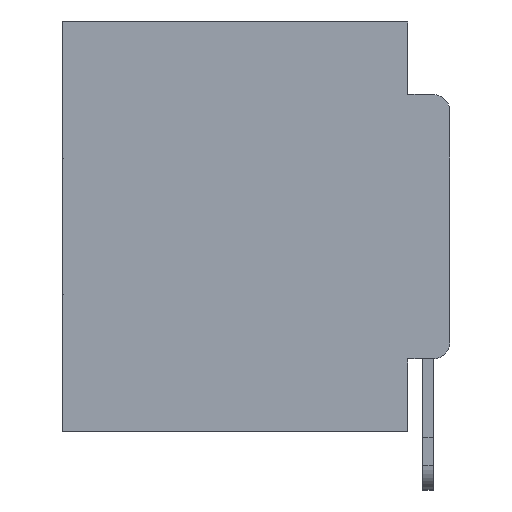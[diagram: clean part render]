
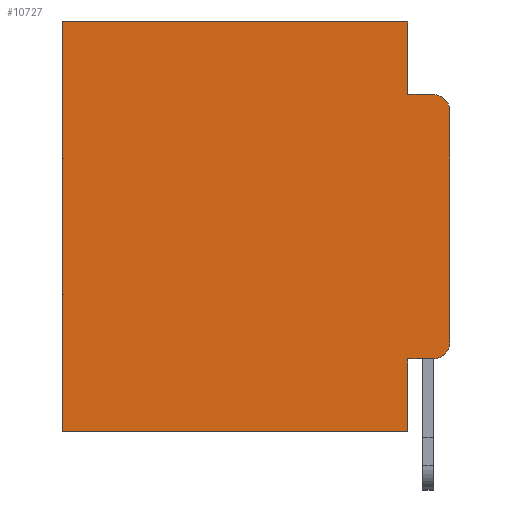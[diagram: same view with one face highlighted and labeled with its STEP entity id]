
A CAD part, left-side view. The second image highlights one B-rep face of the part: STEP entity #10727.
In plain terms, the highlighted planar face has unit normal (-1, 0, 0).
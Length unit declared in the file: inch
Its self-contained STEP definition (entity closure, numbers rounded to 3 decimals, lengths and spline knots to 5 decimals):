
#312 = CARTESIAN_POINT ( 'NONE',  ( 0.298, 0., -0.5 ) ) ;
#399 = EDGE_CURVE ( 'NONE', #8756, #29636, #10669, .T. ) ;
#598 = CARTESIAN_POINT ( 'NONE',  ( 0.298, 0.051, -0.5 ) ) ;
#694 = VERTEX_POINT ( 'NONE', #23454 ) ;
#695 = CARTESIAN_POINT ( 'NONE',  ( 0.298, 0.051, -0.0885 ) ) ;
#1277 = CARTESIAN_POINT ( 'NONE',  ( 0.298, 0.473, 0. ) ) ;
#1932 = CARTESIAN_POINT ( 'NONE',  ( 0.298, 0., -0.3915 ) ) ;
#1965 = ORIENTED_EDGE ( 'NONE', *, *, #18255, .T. ) ;
#2171 = VERTEX_POINT ( 'NONE', #18730 ) ;
#2199 = VERTEX_POINT ( 'NONE', #28101 ) ;
#2334 = ORIENTED_EDGE ( 'NONE', *, *, #22888, .F. ) ;
#2927 = VERTEX_POINT ( 'NONE', #16836 ) ;
#3115 = DIRECTION ( 'NONE',  ( 0., 1., 0. ) ) ;
#3500 = CARTESIAN_POINT ( 'NONE',  ( 0.298, 0.02, -0.3915 ) ) ;
#3688 = CARTESIAN_POINT ( 'NONE',  ( 0.298, 0.02, -0.4115 ) ) ;
#3962 = EDGE_CURVE ( 'NONE', #8756, #24440, #10182, .T. ) ;
#4555 = VECTOR ( 'NONE', #7029, 39.37008 ) ;
#4608 = ORIENTED_EDGE ( 'NONE', *, *, #13509, .F. ) ;
#5207 = DIRECTION ( 'NONE',  ( 0., 1., 0. ) ) ;
#5324 = VECTOR ( 'NONE', #5207, 39.37008 ) ;
#5729 = DIRECTION ( 'NONE',  ( -1., 0., 0. ) ) ;
#6112 = DIRECTION ( 'NONE',  ( 1., 0., 0. ) ) ;
#6208 = DIRECTION ( 'NONE',  ( 0., 0., -1. ) ) ;
#6570 = DIRECTION ( 'NONE',  ( 0., 0., -1. ) ) ;
#6947 = EDGE_CURVE ( 'NONE', #2199, #2927, #21695, .T. ) ;
#7029 = DIRECTION ( 'NONE',  ( 0., -1., 0. ) ) ;
#7343 = DIRECTION ( 'NONE',  ( -1., 0., 0. ) ) ;
#7470 = LINE ( 'NONE', #26134, #7852 ) ;
#7674 = LINE ( 'NONE', #20379, #8401 ) ;
#7852 = VECTOR ( 'NONE', #3115, 39.37008 ) ;
#8401 = VECTOR ( 'NONE', #6570, 39.37008 ) ;
#8756 = VERTEX_POINT ( 'NONE', #10710 ) ;
#8997 = ORIENTED_EDGE ( 'NONE', *, *, #399, .T. ) ;
#9087 = ORIENTED_EDGE ( 'NONE', *, *, #18671, .F. ) ;
#9179 = VERTEX_POINT ( 'NONE', #1932 ) ;
#10135 = VERTEX_POINT ( 'NONE', #695 ) ;
#10182 = LINE ( 'NONE', #28171, #19637 ) ;
#10669 = LINE ( 'NONE', #27706, #4555 ) ;
#10710 = CARTESIAN_POINT ( 'NONE',  ( 0.298, 0.051, -0.4115 ) ) ;
#10727 = ADVANCED_FACE ( 'NONE', ( #23800 ), #24559, .F. ) ;
#12196 = DIRECTION ( 'NONE',  ( 0., 0., -1. ) ) ;
#12532 = ORIENTED_EDGE ( 'NONE', *, *, #17677, .T. ) ;
#13153 = VERTEX_POINT ( 'NONE', #1277 ) ;
#13509 = EDGE_CURVE ( 'NONE', #10135, #2927, #26565, .T. ) ;
#14020 = DIRECTION ( 'NONE',  ( 0., 0., -1. ) ) ;
#14524 = VECTOR ( 'NONE', #21145, 39.37008 ) ;
#16315 = DIRECTION ( 'NONE',  ( 0., 0., -1. ) ) ;
#16836 = CARTESIAN_POINT ( 'NONE',  ( 0.298, 0.02, -0.0885 ) ) ;
#17427 = LINE ( 'NONE', #21117, #21453 ) ;
#17677 = EDGE_CURVE ( 'NONE', #13153, #2171, #23354, .T. ) ;
#18255 = EDGE_CURVE ( 'NONE', #29636, #9179, #20411, .T. ) ;
#18609 = DIRECTION ( 'NONE',  ( 0., 0., -1. ) ) ;
#18671 = EDGE_CURVE ( 'NONE', #2199, #9179, #17427, .T. ) ;
#18730 = CARTESIAN_POINT ( 'NONE',  ( 0.298, 0.473, -0.5 ) ) ;
#19408 = EDGE_LOOP ( 'NONE', ( #9087, #23281, #4608, #22141, #21606, #12532, #2334, #27607, #8997, #1965 ) ) ;
#19637 = VECTOR ( 'NONE', #18609, 39.37008 ) ;
#19952 = CARTESIAN_POINT ( 'NONE',  ( 0.298, 0.051, -0.0885 ) ) ;
#20379 = CARTESIAN_POINT ( 'NONE',  ( 0.298, 0.051, 0. ) ) ;
#20411 = CIRCLE ( 'NONE', #23988, 0.02 ) ;
#21117 = CARTESIAN_POINT ( 'NONE',  ( 0.298, 0., 0. ) ) ;
#21145 = DIRECTION ( 'NONE',  ( 0., -1., 0. ) ) ;
#21453 = VECTOR ( 'NONE', #16315, 39.37008 ) ;
#21606 = ORIENTED_EDGE ( 'NONE', *, *, #22400, .T. ) ;
#21695 = CIRCLE ( 'NONE', #27188, 0.02 ) ;
#21758 = DIRECTION ( 'NONE',  ( 0., 0., -1. ) ) ;
#21894 = VECTOR ( 'NONE', #12196, 39.37008 ) ;
#22141 = ORIENTED_EDGE ( 'NONE', *, *, #27830, .F. ) ;
#22400 = EDGE_CURVE ( 'NONE', #694, #13153, #7470, .T. ) ;
#22888 = EDGE_CURVE ( 'NONE', #24440, #2171, #23458, .T. ) ;
#23281 = ORIENTED_EDGE ( 'NONE', *, *, #6947, .T. ) ;
#23354 = LINE ( 'NONE', #28270, #21894 ) ;
#23454 = CARTESIAN_POINT ( 'NONE',  ( 0.298, 0.051, 0. ) ) ;
#23458 = LINE ( 'NONE', #312, #5324 ) ;
#23800 = FACE_OUTER_BOUND ( 'NONE', #19408, .T. ) ;
#23988 = AXIS2_PLACEMENT_3D ( 'NONE', #3500, #5729, #21758 ) ;
#24440 = VERTEX_POINT ( 'NONE', #598 ) ;
#24559 = PLANE ( 'NONE',  #27289 ) ;
#26134 = CARTESIAN_POINT ( 'NONE',  ( 0.298, 0., 0. ) ) ;
#26565 = LINE ( 'NONE', #19952, #14524 ) ;
#27188 = AXIS2_PLACEMENT_3D ( 'NONE', #27989, #7343, #14020 ) ;
#27289 = AXIS2_PLACEMENT_3D ( 'NONE', #29240, #6112, #6208 ) ;
#27607 = ORIENTED_EDGE ( 'NONE', *, *, #3962, .F. ) ;
#27706 = CARTESIAN_POINT ( 'NONE',  ( 0.298, 0.051, -0.4115 ) ) ;
#27830 = EDGE_CURVE ( 'NONE', #694, #10135, #7674, .T. ) ;
#27989 = CARTESIAN_POINT ( 'NONE',  ( 0.298, 0.02, -0.1085 ) ) ;
#28101 = CARTESIAN_POINT ( 'NONE',  ( 0.298, 0., -0.1085 ) ) ;
#28171 = CARTESIAN_POINT ( 'NONE',  ( 0.298, 0.051, 0. ) ) ;
#28270 = CARTESIAN_POINT ( 'NONE',  ( 0.298, 0.473, 0. ) ) ;
#29240 = CARTESIAN_POINT ( 'NONE',  ( 0.298, 0., 0. ) ) ;
#29636 = VERTEX_POINT ( 'NONE', #3688 ) ;
